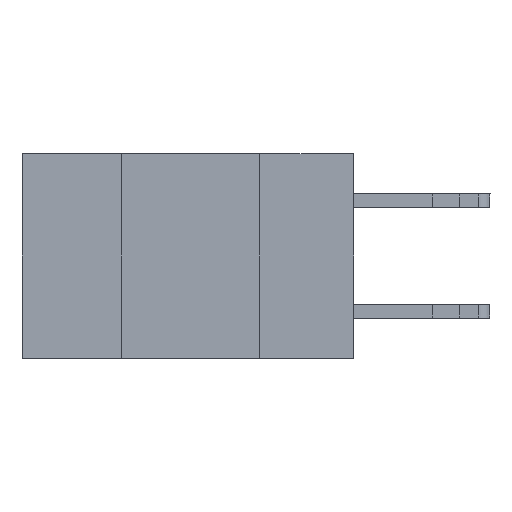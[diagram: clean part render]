
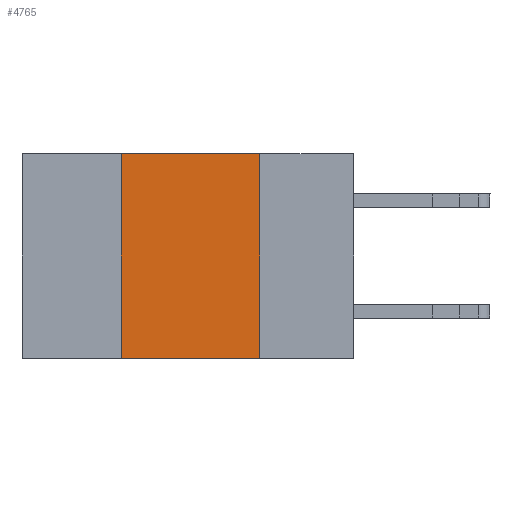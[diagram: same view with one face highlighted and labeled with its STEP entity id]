
A CAD part, left-side view. The second image highlights one B-rep face of the part: STEP entity #4765.
In plain terms, the highlighted planar face has unit normal (-1, 0, 0).
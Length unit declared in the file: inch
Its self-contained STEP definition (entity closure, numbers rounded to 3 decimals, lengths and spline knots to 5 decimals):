
#68 = EDGE_CURVE ( 'NONE', #26151, #25023, #14154, .T. ) ;
#2396 = DIRECTION ( 'NONE',  ( 0., 0., 1. ) ) ;
#3492 = CARTESIAN_POINT ( 'NONE',  ( 0., 0.6, 0. ) ) ;
#4598 = DIRECTION ( 'NONE',  ( 0., 0., -1. ) ) ;
#4638 = ORIENTED_EDGE ( 'NONE', *, *, #20569, .T. ) ;
#4722 = LINE ( 'NONE', #9908, #19730 ) ;
#4765 = ADVANCED_FACE ( 'NONE', ( #12391 ), #9892, .F. ) ;
#5553 = VERTEX_POINT ( 'NONE', #8177 ) ;
#6406 = CARTESIAN_POINT ( 'NONE',  ( 0., 0.17, 0. ) ) ;
#6416 = ORIENTED_EDGE ( 'NONE', *, *, #27595, .F. ) ;
#7114 = CARTESIAN_POINT ( 'NONE',  ( 0., 0.17, 0. ) ) ;
#8177 = CARTESIAN_POINT ( 'NONE',  ( 0., 0.17, -0.37 ) ) ;
#9892 = PLANE ( 'NONE',  #22059 ) ;
#9908 = CARTESIAN_POINT ( 'NONE',  ( 0., 0.42, 0. ) ) ;
#11079 = DIRECTION ( 'NONE',  ( 0., -1., 0. ) ) ;
#12391 = FACE_OUTER_BOUND ( 'NONE', #22252, .T. ) ;
#12988 = VECTOR ( 'NONE', #13988, 39.37008 ) ;
#13575 = LINE ( 'NONE', #20888, #31115 ) ;
#13988 = DIRECTION ( 'NONE',  ( 0., -1., 0. ) ) ;
#14154 = LINE ( 'NONE', #3492, #12988 ) ;
#15538 = CARTESIAN_POINT ( 'NONE',  ( 0., 0.42, -0.37 ) ) ;
#17547 = DIRECTION ( 'NONE',  ( 0., 0., -1. ) ) ;
#19068 = VERTEX_POINT ( 'NONE', #15538 ) ;
#19730 = VECTOR ( 'NONE', #2396, 39.37008 ) ;
#20569 = EDGE_CURVE ( 'NONE', #19068, #5553, #13575, .T. ) ;
#20784 = VECTOR ( 'NONE', #4598, 39.37008 ) ;
#20888 = CARTESIAN_POINT ( 'NONE',  ( 0., 0.6, -0.37 ) ) ;
#21097 = CARTESIAN_POINT ( 'NONE',  ( 0., 0.42, 0. ) ) ;
#21997 = ORIENTED_EDGE ( 'NONE', *, *, #68, .F. ) ;
#22059 = AXIS2_PLACEMENT_3D ( 'NONE', #32290, #31969, #17547 ) ;
#22252 = EDGE_LOOP ( 'NONE', ( #6416, #21997, #30746, #4638 ) ) ;
#25023 = VERTEX_POINT ( 'NONE', #6406 ) ;
#26151 = VERTEX_POINT ( 'NONE', #21097 ) ;
#27595 = EDGE_CURVE ( 'NONE', #25023, #5553, #29851, .T. ) ;
#28126 = EDGE_CURVE ( 'NONE', #19068, #26151, #4722, .T. ) ;
#29851 = LINE ( 'NONE', #7114, #20784 ) ;
#30746 = ORIENTED_EDGE ( 'NONE', *, *, #28126, .F. ) ;
#31115 = VECTOR ( 'NONE', #11079, 39.37008 ) ;
#31969 = DIRECTION ( 'NONE',  ( 1., 0., 0. ) ) ;
#32290 = CARTESIAN_POINT ( 'NONE',  ( 0., 0.6, 0. ) ) ;
